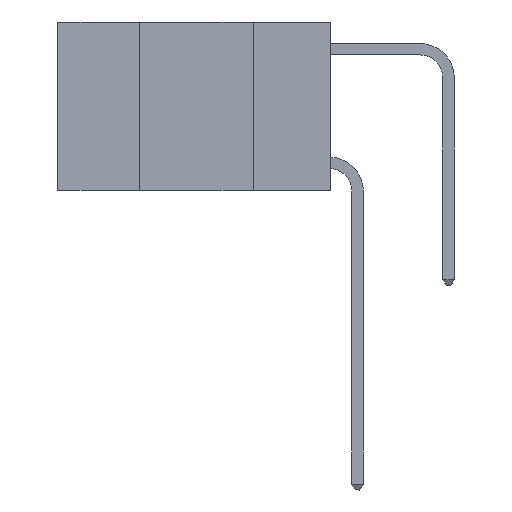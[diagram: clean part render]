
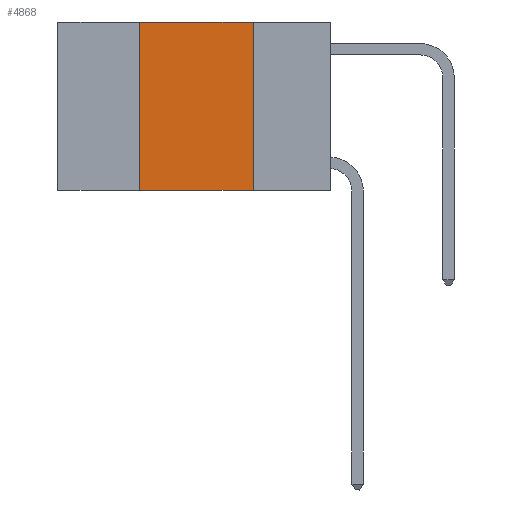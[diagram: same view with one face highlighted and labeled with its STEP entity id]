
A CAD part, left-side view. The second image highlights one B-rep face of the part: STEP entity #4868.
In plain terms, the highlighted planar face has unit normal (-1, 0, 0).
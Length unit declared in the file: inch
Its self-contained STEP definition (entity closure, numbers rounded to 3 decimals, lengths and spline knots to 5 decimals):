
#338 = PLANE ( 'NONE',  #8580 ) ;
#406 = CARTESIAN_POINT ( 'NONE',  ( 0., 0.6, 0. ) ) ;
#429 = DIRECTION ( 'NONE',  ( 0., 0., -1. ) ) ;
#554 = CARTESIAN_POINT ( 'NONE',  ( 0., 0.42, 0. ) ) ;
#867 = VERTEX_POINT ( 'NONE', #17314 ) ;
#972 = CARTESIAN_POINT ( 'NONE',  ( 0., 0.6, -0.37 ) ) ;
#1371 = LINE ( 'NONE', #406, #21601 ) ;
#2384 = LINE ( 'NONE', #554, #6976 ) ;
#2894 = ORIENTED_EDGE ( 'NONE', *, *, #10642, .F. ) ;
#4868 = ADVANCED_FACE ( 'NONE', ( #15734 ), #338, .F. ) ;
#6976 = VECTOR ( 'NONE', #22081, 39.37008 ) ;
#7270 = CARTESIAN_POINT ( 'NONE',  ( 0., 0.17, 0. ) ) ;
#8580 = AXIS2_PLACEMENT_3D ( 'NONE', #14068, #12192, #429 ) ;
#8739 = ORIENTED_EDGE ( 'NONE', *, *, #21866, .F. ) ;
#9594 = EDGE_CURVE ( 'NONE', #867, #21795, #19484, .T. ) ;
#10642 = EDGE_CURVE ( 'NONE', #18253, #19650, #1371, .T. ) ;
#10939 = VECTOR ( 'NONE', #22491, 39.37008 ) ;
#12192 = DIRECTION ( 'NONE',  ( 1., 0., 0. ) ) ;
#13381 = CARTESIAN_POINT ( 'NONE',  ( 0., 0.42, 0. ) ) ;
#13944 = ORIENTED_EDGE ( 'NONE', *, *, #9594, .T. ) ;
#14068 = CARTESIAN_POINT ( 'NONE',  ( 0., 0.6, 0. ) ) ;
#15409 = VECTOR ( 'NONE', #22955, 39.37008 ) ;
#15734 = FACE_OUTER_BOUND ( 'NONE', #17659, .T. ) ;
#15994 = LINE ( 'NONE', #7270, #15409 ) ;
#17314 = CARTESIAN_POINT ( 'NONE',  ( 0., 0.42, -0.37 ) ) ;
#17659 = EDGE_LOOP ( 'NONE', ( #23158, #2894, #8739, #13944 ) ) ;
#18253 = VERTEX_POINT ( 'NONE', #13381 ) ;
#18751 = EDGE_CURVE ( 'NONE', #19650, #21795, #15994, .T. ) ;
#19484 = LINE ( 'NONE', #972, #10939 ) ;
#19630 = CARTESIAN_POINT ( 'NONE',  ( 0., 0.17, 0. ) ) ;
#19650 = VERTEX_POINT ( 'NONE', #19630 ) ;
#20051 = DIRECTION ( 'NONE',  ( 0., -1., 0. ) ) ;
#21601 = VECTOR ( 'NONE', #20051, 39.37008 ) ;
#21795 = VERTEX_POINT ( 'NONE', #21909 ) ;
#21866 = EDGE_CURVE ( 'NONE', #867, #18253, #2384, .T. ) ;
#21909 = CARTESIAN_POINT ( 'NONE',  ( 0., 0.17, -0.37 ) ) ;
#22081 = DIRECTION ( 'NONE',  ( 0., 0., 1. ) ) ;
#22491 = DIRECTION ( 'NONE',  ( 0., -1., 0. ) ) ;
#22955 = DIRECTION ( 'NONE',  ( 0., 0., -1. ) ) ;
#23158 = ORIENTED_EDGE ( 'NONE', *, *, #18751, .F. ) ;
